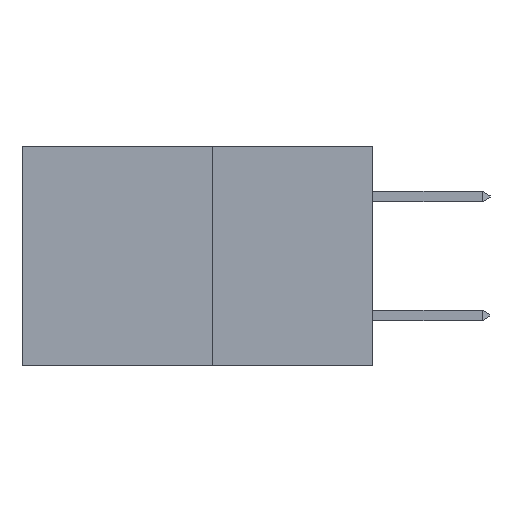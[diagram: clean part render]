
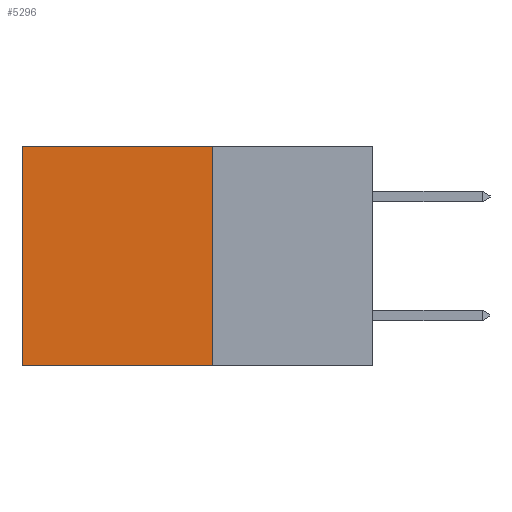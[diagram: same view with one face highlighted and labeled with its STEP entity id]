
A CAD part, left-side view. The second image highlights one B-rep face of the part: STEP entity #5296.
In plain terms, the highlighted planar face has unit normal (-1, 0, 0).
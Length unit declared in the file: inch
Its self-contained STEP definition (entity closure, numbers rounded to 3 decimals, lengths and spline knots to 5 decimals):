
#186 = FACE_OUTER_BOUND ( 'NONE', #317, .T. ) ;
#317 = EDGE_LOOP ( 'NONE', ( #3938, #24018, #6346, #22725 ) ) ;
#1181 = VERTEX_POINT ( 'NONE', #25896 ) ;
#1480 = VECTOR ( 'NONE', #27629, 39.37008 ) ;
#2739 = CARTESIAN_POINT ( 'NONE',  ( 0.277, 0.59, 0. ) ) ;
#2757 = VECTOR ( 'NONE', #28397, 39.37008 ) ;
#2848 = LINE ( 'NONE', #3307, #1480 ) ;
#3307 = CARTESIAN_POINT ( 'NONE',  ( 0.277, 0.27, 0. ) ) ;
#3938 = ORIENTED_EDGE ( 'NONE', *, *, #22632, .T. ) ;
#4276 = LINE ( 'NONE', #27737, #27088 ) ;
#5259 = VERTEX_POINT ( 'NONE', #28209 ) ;
#5296 = ADVANCED_FACE ( 'NONE', ( #186 ), #6280, .F. ) ;
#6280 = PLANE ( 'NONE',  #19380 ) ;
#6346 = ORIENTED_EDGE ( 'NONE', *, *, #11552, .F. ) ;
#6534 = CARTESIAN_POINT ( 'NONE',  ( 0.277, 0.27, -0.37 ) ) ;
#7155 = EDGE_CURVE ( 'NONE', #21510, #5259, #4276, .T. ) ;
#8477 = DIRECTION ( 'NONE',  ( 0., 0., -1. ) ) ;
#10527 = LINE ( 'NONE', #25221, #27466 ) ;
#11552 = EDGE_CURVE ( 'NONE', #1181, #21510, #10527, .T. ) ;
#12855 = CARTESIAN_POINT ( 'NONE',  ( 0.277, 0.27, -0.37 ) ) ;
#14119 = DIRECTION ( 'NONE',  ( 0., 0., -1. ) ) ;
#16557 = LINE ( 'NONE', #19526, #2757 ) ;
#16784 = VERTEX_POINT ( 'NONE', #2739 ) ;
#19380 = AXIS2_PLACEMENT_3D ( 'NONE', #12855, #21735, #8477 ) ;
#19526 = CARTESIAN_POINT ( 'NONE',  ( 0.277, 0.59, -0.37 ) ) ;
#21077 = DIRECTION ( 'NONE',  ( 0., 1., 0. ) ) ;
#21510 = VERTEX_POINT ( 'NONE', #6534 ) ;
#21735 = DIRECTION ( 'NONE',  ( 1., 0., 0. ) ) ;
#22632 = EDGE_CURVE ( 'NONE', #16784, #5259, #16557, .T. ) ;
#22725 = ORIENTED_EDGE ( 'NONE', *, *, #25987, .T. ) ;
#24018 = ORIENTED_EDGE ( 'NONE', *, *, #7155, .F. ) ;
#25221 = CARTESIAN_POINT ( 'NONE',  ( 0.277, 0.27, -0.37 ) ) ;
#25896 = CARTESIAN_POINT ( 'NONE',  ( 0.277, 0.27, 0. ) ) ;
#25987 = EDGE_CURVE ( 'NONE', #1181, #16784, #2848, .T. ) ;
#27088 = VECTOR ( 'NONE', #21077, 39.37008 ) ;
#27466 = VECTOR ( 'NONE', #14119, 39.37008 ) ;
#27629 = DIRECTION ( 'NONE',  ( 0., 1., 0. ) ) ;
#27737 = CARTESIAN_POINT ( 'NONE',  ( 0.277, 0.27, -0.37 ) ) ;
#28209 = CARTESIAN_POINT ( 'NONE',  ( 0.277, 0.59, -0.37 ) ) ;
#28397 = DIRECTION ( 'NONE',  ( 0., 0., -1. ) ) ;
